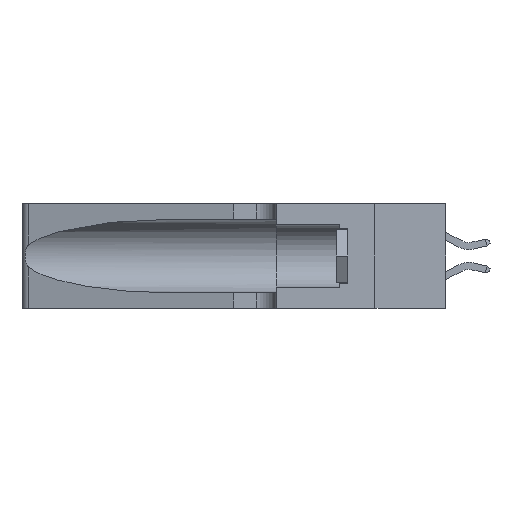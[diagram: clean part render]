
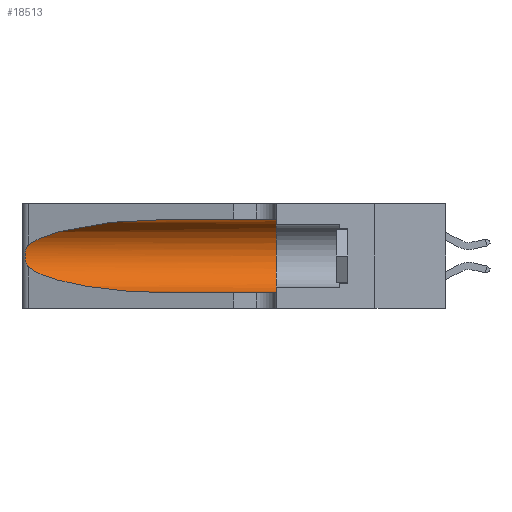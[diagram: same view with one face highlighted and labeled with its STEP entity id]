
A CAD part, left-side view. The second image highlights one B-rep face of the part: STEP entity #18513.
In plain terms, the highlighted cylindrical face has radius 3.308 mm (diameter 6.617 mm), a partial arc.
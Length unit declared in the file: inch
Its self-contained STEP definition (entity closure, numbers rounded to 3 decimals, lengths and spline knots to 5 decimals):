
#93 = EDGE_CURVE ( 'NONE', #20779, #11105, #2277, .T. ) ;
#506 = CARTESIAN_POINT ( 'NONE',  ( 0.26017, 1.23833, 0.17102 ) ) ;
#658 = CYLINDRICAL_SURFACE ( 'NONE', #2705, 0.13025 ) ;
#962 = CARTESIAN_POINT ( 'NONE',  ( 0.1305, 0.72297, 0.05475 ) ) ;
#1285 = CARTESIAN_POINT ( 'NONE',  ( 0.1305, 1.61858, 0.185 ) ) ;
#1583 = CARTESIAN_POINT ( 'NONE',  ( 0.18966, 0.96281, 0.31525 ) ) ;
#1917 = CARTESIAN_POINT ( 'NONE',  ( 0.1305, 0.72297, 0.31525 ) ) ;
#2072 = CARTESIAN_POINT ( 'NONE',  ( 0.1305, 0.72297, 0.31525 ) ) ;
#2277 =( BOUNDED_CURVE ( )  B_SPLINE_CURVE ( 3, ( #1917, #1583, #6927, #14271 ),
 .UNSPECIFIED., .F., .T. ) 
 B_SPLINE_CURVE_WITH_KNOTS ( ( 4, 4 ),
 ( 1.5708, 2.84003 ),
 .UNSPECIFIED. ) 
 CURVE ( )  GEOMETRIC_REPRESENTATION_ITEM ( )  RATIONAL_B_SPLINE_CURVE ( ( 1., 0.87, 0.87, 1. ) ) 
 REPRESENTATION_ITEM ( '' )  );
#2376 = CARTESIAN_POINT ( 'NONE',  ( 0.25555, 1.22994, 0.2215 ) ) ;
#2452 = CARTESIAN_POINT ( 'NONE',  ( 0.25789, 1.23486, 0.15765 ) ) ;
#2613 = EDGE_LOOP ( 'NONE', ( #7982, #12797, #3719, #18756, #5411, #10946 ) ) ;
#2705 = AXIS2_PLACEMENT_3D ( 'NONE', #1285, #14086, #12262 ) ;
#2717 = DIRECTION ( 'NONE',  ( 0., -1., 0. ) ) ;
#3719 = ORIENTED_EDGE ( 'NONE', *, *, #16000, .T. ) ;
#4286 = CARTESIAN_POINT ( 'NONE',  ( 0.25555, 1.22993, 0.14849 ) ) ;
#4663 = VERTEX_POINT ( 'NONE', #13929 ) ;
#5010 = VECTOR ( 'NONE', #2717, 39.37008 ) ;
#5411 = ORIENTED_EDGE ( 'NONE', *, *, #15201, .F. ) ;
#5673 = DIRECTION ( 'NONE',  ( 0., 1., 0. ) ) ;
#6303 = CARTESIAN_POINT ( 'NONE',  ( 0.25487, 1.22718, 0.14631 ) ) ;
#6664 = VECTOR ( 'NONE', #13102, 39.37008 ) ;
#6762 = CARTESIAN_POINT ( 'NONE',  ( 0.1305, 0.35, 0.05475 ) ) ;
#6927 = CARTESIAN_POINT ( 'NONE',  ( 0.2373, 1.15595, 0.28018 ) ) ;
#7320 = CARTESIAN_POINT ( 'NONE',  ( 0.25487, 1.22718, 0.22369 ) ) ;
#7714 = CARTESIAN_POINT ( 'NONE',  ( 0.1305, 1.61858, 0.05475 ) ) ;
#7876 = CARTESIAN_POINT ( 'NONE',  ( 0.25787, 1.23484, 0.2124 ) ) ;
#7982 = ORIENTED_EDGE ( 'NONE', *, *, #93, .T. ) ;
#8116 = CARTESIAN_POINT ( 'NONE',  ( 0.18966, 0.96281, 0.05475 ) ) ;
#8278 = VERTEX_POINT ( 'NONE', #20466 ) ;
#9423 =( BOUNDED_CURVE ( )  B_SPLINE_CURVE ( 3, ( #6303, #17186, #8116, #20807 ),
 .UNSPECIFIED., .F., .F. ) 
 B_SPLINE_CURVE_WITH_KNOTS ( ( 4, 4 ),
 ( 3.44316, 4.71239 ),
 .UNSPECIFIED. ) 
 CURVE ( )  GEOMETRIC_REPRESENTATION_ITEM ( )  RATIONAL_B_SPLINE_CURVE ( ( 1., 0.87, 0.87, 1. ) ) 
 REPRESENTATION_ITEM ( '' )  );
#9681 = CARTESIAN_POINT ( 'NONE',  ( 0.26018, 1.23835, 0.19895 ) ) ;
#10946 = ORIENTED_EDGE ( 'NONE', *, *, #19018, .F. ) ;
#11105 = VERTEX_POINT ( 'NONE', #7320 ) ;
#11517 = CARTESIAN_POINT ( 'NONE',  ( 0.26075, 1.23896, 0.178 ) ) ;
#11897 = B_SPLINE_CURVE_WITH_KNOTS ( 'NONE', 3,
 ( #15081, #2376, #18732, #7876, #20554, #9681, #22357, #11517, #506, #13342, #2452, #15157, #4286, #17013 ),
 .UNSPECIFIED., .F., .F.,
 ( 4, 2, 2, 2, 2, 2, 4 ),
 ( 0., 0.00027, 0.00053, 0.00107, 0.0016, 0.00187, 0.00214 ),
 .UNSPECIFIED. ) ;
#12065 = LINE ( 'NONE', #7714, #6664 ) ;
#12262 = DIRECTION ( 'NONE',  ( 0., 0., -1. ) ) ;
#12797 = ORIENTED_EDGE ( 'NONE', *, *, #21514, .T. ) ;
#13102 = DIRECTION ( 'NONE',  ( 0., -1., 0. ) ) ;
#13267 = EDGE_CURVE ( 'NONE', #13482, #16187, #12065, .T. ) ;
#13342 = CARTESIAN_POINT ( 'NONE',  ( 0.25856, 1.23593, 0.16098 ) ) ;
#13482 = VERTEX_POINT ( 'NONE', #962 ) ;
#13773 = AXIS2_PLACEMENT_3D ( 'NONE', #16594, #5673, #18389 ) ;
#13929 = CARTESIAN_POINT ( 'NONE',  ( 0.25487, 1.22718, 0.14631 ) ) ;
#14086 = DIRECTION ( 'NONE',  ( 0., -1., 0. ) ) ;
#14110 = LINE ( 'NONE', #15405, #5010 ) ;
#14271 = CARTESIAN_POINT ( 'NONE',  ( 0.25487, 1.22718, 0.22369 ) ) ;
#15081 = CARTESIAN_POINT ( 'NONE',  ( 0.25487, 1.22718, 0.22369 ) ) ;
#15157 = CARTESIAN_POINT ( 'NONE',  ( 0.25639, 1.23186, 0.15144 ) ) ;
#15201 = EDGE_CURVE ( 'NONE', #8278, #16187, #18835, .T. ) ;
#15259 = FACE_OUTER_BOUND ( 'NONE', #2613, .T. ) ;
#15405 = CARTESIAN_POINT ( 'NONE',  ( 0.1305, 1.61858, 0.31525 ) ) ;
#16000 = EDGE_CURVE ( 'NONE', #4663, #13482, #9423, .T. ) ;
#16187 = VERTEX_POINT ( 'NONE', #6762 ) ;
#16594 = CARTESIAN_POINT ( 'NONE',  ( 0.1305, 0.35, 0.185 ) ) ;
#17013 = CARTESIAN_POINT ( 'NONE',  ( 0.25487, 1.22718, 0.14631 ) ) ;
#17186 = CARTESIAN_POINT ( 'NONE',  ( 0.2373, 1.15595, 0.08982 ) ) ;
#18389 = DIRECTION ( 'NONE',  ( 0., 0., 1. ) ) ;
#18513 = ADVANCED_FACE ( 'NONE', ( #15259 ), #658, .F. ) ;
#18732 = CARTESIAN_POINT ( 'NONE',  ( 0.25639, 1.23184, 0.21858 ) ) ;
#18756 = ORIENTED_EDGE ( 'NONE', *, *, #13267, .T. ) ;
#18835 = CIRCLE ( 'NONE', #13773, 0.13025 ) ;
#19018 = EDGE_CURVE ( 'NONE', #20779, #8278, #14110, .T. ) ;
#20466 = CARTESIAN_POINT ( 'NONE',  ( 0.1305, 0.35, 0.31525 ) ) ;
#20554 = CARTESIAN_POINT ( 'NONE',  ( 0.25854, 1.2359, 0.20912 ) ) ;
#20779 = VERTEX_POINT ( 'NONE', #2072 ) ;
#20807 = CARTESIAN_POINT ( 'NONE',  ( 0.1305, 0.72297, 0.05475 ) ) ;
#21514 = EDGE_CURVE ( 'NONE', #11105, #4663, #11897, .T. ) ;
#22357 = CARTESIAN_POINT ( 'NONE',  ( 0.26075, 1.23896, 0.19203 ) ) ;
